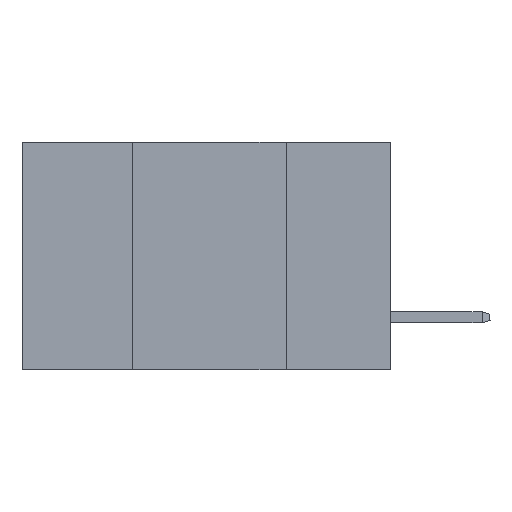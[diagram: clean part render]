
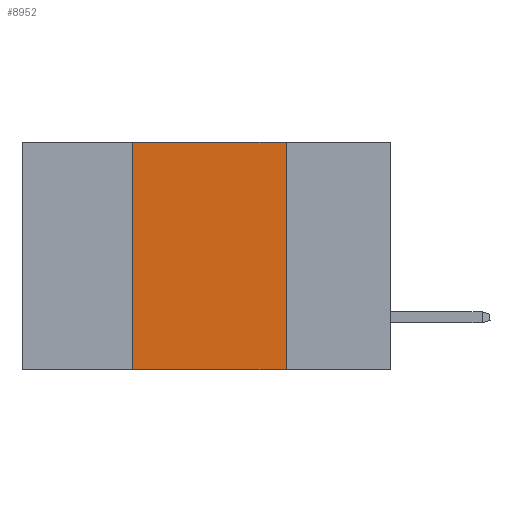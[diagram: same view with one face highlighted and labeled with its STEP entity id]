
A CAD part, left-side view. The second image highlights one B-rep face of the part: STEP entity #8952.
In plain terms, the highlighted planar face has unit normal (-1, 0, 0).
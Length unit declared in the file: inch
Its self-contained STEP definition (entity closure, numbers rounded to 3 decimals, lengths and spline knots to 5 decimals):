
#663 = EDGE_CURVE ( 'NONE', #39312, #19660, #14665, .T. ) ;
#1465 = CARTESIAN_POINT ( 'NONE',  ( 0., 0.6, 0. ) ) ;
#2014 = ORIENTED_EDGE ( 'NONE', *, *, #20197, .F. ) ;
#2924 = DIRECTION ( 'NONE',  ( 0., 0., 1. ) ) ;
#3018 = AXIS2_PLACEMENT_3D ( 'NONE', #19160, #19467, #36523 ) ;
#4171 = EDGE_LOOP ( 'NONE', ( #26092, #2014, #18193, #33703 ) ) ;
#4937 = CARTESIAN_POINT ( 'NONE',  ( 0., 0.17, -0.37 ) ) ;
#5554 = PLANE ( 'NONE',  #3018 ) ;
#7009 = VERTEX_POINT ( 'NONE', #15800 ) ;
#7401 = CARTESIAN_POINT ( 'NONE',  ( 0., 0.6, -0.37 ) ) ;
#7453 = CARTESIAN_POINT ( 'NONE',  ( 0., 0.42, -0.37 ) ) ;
#8223 = EDGE_CURVE ( 'NONE', #7009, #42474, #37613, .T. ) ;
#8952 = ADVANCED_FACE ( 'NONE', ( #28240 ), #5554, .F. ) ;
#8988 = DIRECTION ( 'NONE',  ( 0., 0., -1. ) ) ;
#10914 = VECTOR ( 'NONE', #39476, 39.37008 ) ;
#11376 = VECTOR ( 'NONE', #31421, 39.37008 ) ;
#14665 = LINE ( 'NONE', #16812, #33307 ) ;
#15402 = CARTESIAN_POINT ( 'NONE',  ( 0., 0.17, 0. ) ) ;
#15800 = CARTESIAN_POINT ( 'NONE',  ( 0., 0.17, 0. ) ) ;
#16812 = CARTESIAN_POINT ( 'NONE',  ( 0., 0.42, 0. ) ) ;
#18193 = ORIENTED_EDGE ( 'NONE', *, *, #663, .F. ) ;
#19160 = CARTESIAN_POINT ( 'NONE',  ( 0., 0.6, 0. ) ) ;
#19467 = DIRECTION ( 'NONE',  ( 1., 0., 0. ) ) ;
#19474 = VECTOR ( 'NONE', #8988, 39.37008 ) ;
#19660 = VERTEX_POINT ( 'NONE', #19934 ) ;
#19934 = CARTESIAN_POINT ( 'NONE',  ( 0., 0.42, 0. ) ) ;
#20197 = EDGE_CURVE ( 'NONE', #19660, #7009, #41155, .T. ) ;
#20705 = LINE ( 'NONE', #7401, #11376 ) ;
#26092 = ORIENTED_EDGE ( 'NONE', *, *, #8223, .F. ) ;
#28240 = FACE_OUTER_BOUND ( 'NONE', #4171, .T. ) ;
#31421 = DIRECTION ( 'NONE',  ( 0., -1., 0. ) ) ;
#33006 = EDGE_CURVE ( 'NONE', #39312, #42474, #20705, .T. ) ;
#33307 = VECTOR ( 'NONE', #2924, 39.37008 ) ;
#33703 = ORIENTED_EDGE ( 'NONE', *, *, #33006, .T. ) ;
#36523 = DIRECTION ( 'NONE',  ( 0., 0., -1. ) ) ;
#37613 = LINE ( 'NONE', #15402, #19474 ) ;
#39312 = VERTEX_POINT ( 'NONE', #7453 ) ;
#39476 = DIRECTION ( 'NONE',  ( 0., -1., 0. ) ) ;
#41155 = LINE ( 'NONE', #1465, #10914 ) ;
#42474 = VERTEX_POINT ( 'NONE', #4937 ) ;
